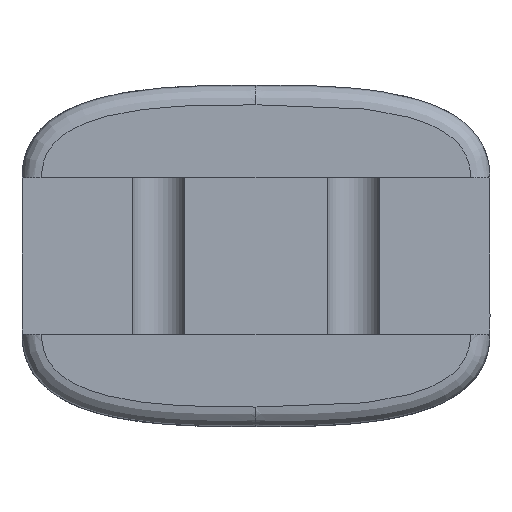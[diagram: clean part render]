
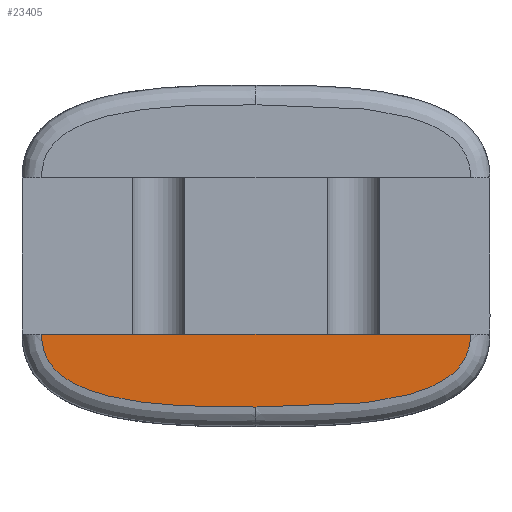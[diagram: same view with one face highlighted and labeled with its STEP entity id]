
A CAD part, top view. The second image highlights one B-rep face of the part: STEP entity #23405.
In plain terms, the highlighted planar face has unit normal (0, 0, 1).
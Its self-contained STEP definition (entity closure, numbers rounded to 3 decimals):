
#26 = CARTESIAN_POINT ( 'NONE',  ( 20.801, 31.551, 43.202 ) ) ;
#451 = CARTESIAN_POINT ( 'NONE',  ( 0., 27.499, 43.202 ) ) ;
#1950 = CARTESIAN_POINT ( 'NONE',  ( -21.732, 33.176, 43.202 ) ) ;
#2040 = CARTESIAN_POINT ( 'NONE',  ( -16.279, 28.948, 43.202 ) ) ;
#2088 = CARTESIAN_POINT ( 'NONE',  ( 14.739, 28.511, 43.202 ) ) ;
#2142 = CARTESIAN_POINT ( 'NONE',  ( 0., 27.499, 43.202 ) ) ;
#2191 = CARTESIAN_POINT ( 'NONE',  ( 21.277, 32.198, 43.202 ) ) ;
#2438 = DIRECTION ( 'NONE',  ( -1., 0., 0. ) ) ;
#3012 = VERTEX_POINT ( 'NONE', #7062 ) ;
#3443 = VERTEX_POINT ( 'NONE', #12315 ) ;
#3592 = CARTESIAN_POINT ( 'NONE',  ( 1.058, 27.499, 43.202 ) ) ;
#3852 = EDGE_CURVE ( 'NONE', #23555, #3012, #21742, .T. ) ;
#4094 = CARTESIAN_POINT ( 'NONE',  ( -21.416, 32.439, 43.202 ) ) ;
#4183 = CARTESIAN_POINT ( 'NONE',  ( -14.744, 28.533, 43.202 ) ) ;
#4212 = ORIENTED_EDGE ( 'NONE', *, *, #3852, .T. ) ;
#4233 = CARTESIAN_POINT ( 'NONE',  ( 16.773, 29.108, 43.202 ) ) ;
#4324 = CARTESIAN_POINT ( 'NONE',  ( 21.634, 32.908, 43.202 ) ) ;
#6139 = ORIENTED_EDGE ( 'NONE', *, *, #10730, .T. ) ;
#6226 = CARTESIAN_POINT ( 'NONE',  ( -20.983, 31.773, 43.202 ) ) ;
#6318 = CARTESIAN_POINT ( 'NONE',  ( -13.187, 28.218, 43.202 ) ) ;
#6364 = CARTESIAN_POINT ( 'NONE',  ( 18.248, 29.703, 43.202 ) ) ;
#6469 = CARTESIAN_POINT ( 'NONE',  ( 21.938, 33.923, 43.202 ) ) ;
#7062 = CARTESIAN_POINT ( 'NONE',  ( 22., 34.963, 43.202 ) ) ;
#8382 = CARTESIAN_POINT ( 'NONE',  ( -20.446, 31.177, 43.202 ) ) ;
#8429 = CARTESIAN_POINT ( 'NONE',  ( 4.23, 27.513, 43.202 ) ) ;
#8481 = CARTESIAN_POINT ( 'NONE',  ( -10.573, 27.849, 43.202 ) ) ;
#8525 = CARTESIAN_POINT ( 'NONE',  ( 19.18, 30.217, 43.202 ) ) ;
#8616 = CARTESIAN_POINT ( 'NONE',  ( 22., 34.963, 43.202 ) ) ;
#10380 = LINE ( 'NONE', #17290, #21672 ) ;
#10497 = CARTESIAN_POINT ( 'NONE',  ( -15.226, 26.597, 43.202 ) ) ;
#10505 = CARTESIAN_POINT ( 'NONE',  ( -19.635, 30.496, 43.202 ) ) ;
#10548 = CARTESIAN_POINT ( 'NONE',  ( 7.399, 27.61, 43.202 ) ) ;
#10597 = CARTESIAN_POINT ( 'NONE',  ( -7.408, 27.611, 43.202 ) ) ;
#10646 = CARTESIAN_POINT ( 'NONE',  ( 19.837, 30.661, 43.202 ) ) ;
#10730 = EDGE_CURVE ( 'NONE', #3443, #23555, #14412, .T. ) ;
#12315 = CARTESIAN_POINT ( 'NONE',  ( -22., 34.963, 43.202 ) ) ;
#12542 = CARTESIAN_POINT ( 'NONE',  ( -21.997, 34.441, 43.202 ) ) ;
#12623 = DIRECTION ( 'NONE',  ( 0., 0., -1. ) ) ;
#12631 = CARTESIAN_POINT ( 'NONE',  ( -18.248, 29.703, 43.202 ) ) ;
#12677 = CARTESIAN_POINT ( 'NONE',  ( 10.562, 27.848, 43.202 ) ) ;
#12727 = CARTESIAN_POINT ( 'NONE',  ( -4.234, 27.513, 43.202 ) ) ;
#12778 = CARTESIAN_POINT ( 'NONE',  ( 20.438, 31.17, 43.202 ) ) ;
#14412 = B_SPLINE_CURVE_WITH_KNOTS ( 'NONE', 3,
 ( #26937, #12542, #14667, #1950, #16812, #4094, #18938, #6226, #21078, #8382, #23216, #10505, #25352, #12631, #27480, #14761, #2040, #16904, #4183, #19027, #6318, #21165, #8481, #23307, #10597, #25445, #12727, #27573, #14846, #2142 ),
 .UNSPECIFIED., .F., .F.,
 ( 4, 2, 2, 2, 2, 2, 2, 2, 2, 2, 2, 2, 2, 2, 4 ),
 ( 0., 0.002, 0.002, 0.003, 0.004, 0.005, 0.006, 0.008, 0.009, 0.011, 0.013, 0.016, 0.019, 0.022, 0.025 ),
 .UNSPECIFIED. ) ;
#14667 = CARTESIAN_POINT ( 'NONE',  ( -21.938, 33.929, 43.202 ) ) ;
#14761 = CARTESIAN_POINT ( 'NONE',  ( -16.78, 29.111, 43.202 ) ) ;
#14802 = CARTESIAN_POINT ( 'NONE',  ( 13.705, 28.3, 43.202 ) ) ;
#14846 = CARTESIAN_POINT ( 'NONE',  ( -1.059, 27.499, 43.202 ) ) ;
#14897 = CARTESIAN_POINT ( 'NONE',  ( 20.972, 31.758, 43.202 ) ) ;
#16474 = ORIENTED_EDGE ( 'NONE', *, *, #26401, .T. ) ;
#16812 = CARTESIAN_POINT ( 'NONE',  ( -21.641, 32.923, 43.202 ) ) ;
#16904 = CARTESIAN_POINT ( 'NONE',  ( -15.261, 28.659, 43.202 ) ) ;
#16951 = CARTESIAN_POINT ( 'NONE',  ( 16.266, 28.944, 43.202 ) ) ;
#17049 = CARTESIAN_POINT ( 'NONE',  ( 21.41, 32.428, 43.202 ) ) ;
#17290 = CARTESIAN_POINT ( 'NONE',  ( -15.226, 34.963, 43.202 ) ) ;
#18678 = AXIS2_PLACEMENT_3D ( 'NONE', #10497, #12623, #27474 ) ;
#18938 = CARTESIAN_POINT ( 'NONE',  ( -21.284, 32.209, 43.202 ) ) ;
#19027 = CARTESIAN_POINT ( 'NONE',  ( -13.708, 28.313, 43.202 ) ) ;
#19042 = FACE_OUTER_BOUND ( 'NONE', #21986, .T. ) ;
#19071 = CARTESIAN_POINT ( 'NONE',  ( 17.764, 29.488, 43.202 ) ) ;
#19164 = CARTESIAN_POINT ( 'NONE',  ( 21.727, 33.159, 43.202 ) ) ;
#21078 = CARTESIAN_POINT ( 'NONE',  ( -20.814, 31.566, 43.202 ) ) ;
#21124 = CARTESIAN_POINT ( 'NONE',  ( 2.115, 27.496, 43.202 ) ) ;
#21165 = CARTESIAN_POINT ( 'NONE',  ( -11.622, 27.968, 43.202 ) ) ;
#21217 = CARTESIAN_POINT ( 'NONE',  ( 18.949, 30.081, 43.202 ) ) ;
#21305 = CARTESIAN_POINT ( 'NONE',  ( 21.997, 34.439, 43.202 ) ) ;
#21672 = VECTOR ( 'NONE', #2438, 1000. ) ;
#21742 = B_SPLINE_CURVE_WITH_KNOTS ( 'NONE', 3,
 ( #24758, #3592, #21124, #8429, #23263, #10548, #25405, #12677, #27530, #14802, #2088, #16951, #4233, #19071, #6364, #21217, #8525, #23351, #10646, #25491, #12778, #26, #14897, #2191, #17049, #4324, #19164, #6469, #21305, #8616 ),
 .UNSPECIFIED., .F., .F.,
 ( 4, 2, 2, 2, 2, 2, 2, 2, 2, 2, 2, 2, 2, 2, 4 ),
 ( 0., 0.003, 0.006, 0.01, 0.013, 0.016, 0.017, 0.019, 0.02, 0.021, 0.021, 0.022, 0.023, 0.024, 0.025 ),
 .UNSPECIFIED. ) ;
#21986 = EDGE_LOOP ( 'NONE', ( #4212, #16474, #6139 ) ) ;
#23216 = CARTESIAN_POINT ( 'NONE',  ( -20.25, 30.998, 43.202 ) ) ;
#23263 = CARTESIAN_POINT ( 'NONE',  ( 5.286, 27.532, 43.202 ) ) ;
#23307 = CARTESIAN_POINT ( 'NONE',  ( -8.466, 27.67, 43.202 ) ) ;
#23351 = CARTESIAN_POINT ( 'NONE',  ( 19.623, 30.507, 43.202 ) ) ;
#23405 = ADVANCED_FACE ( 'NONE', ( #19042 ), #25255, .F. ) ;
#23555 = VERTEX_POINT ( 'NONE', #451 ) ;
#24758 = CARTESIAN_POINT ( 'NONE',  ( 0., 27.499, 43.202 ) ) ;
#25255 = PLANE ( 'NONE',  #18678 ) ;
#25352 = CARTESIAN_POINT ( 'NONE',  ( -19.186, 30.208, 43.202 ) ) ;
#25405 = CARTESIAN_POINT ( 'NONE',  ( 8.454, 27.669, 43.202 ) ) ;
#25445 = CARTESIAN_POINT ( 'NONE',  ( -5.292, 27.532, 43.202 ) ) ;
#25491 = CARTESIAN_POINT ( 'NONE',  ( 20.244, 30.992, 43.202 ) ) ;
#26401 = EDGE_CURVE ( 'NONE', #3012, #3443, #10380, .T. ) ;
#26937 = CARTESIAN_POINT ( 'NONE',  ( -22., 34.963, 43.202 ) ) ;
#27474 = DIRECTION ( 'NONE',  ( 0., 1., 0. ) ) ;
#27480 = CARTESIAN_POINT ( 'NONE',  ( -17.765, 29.489, 43.202 ) ) ;
#27530 = CARTESIAN_POINT ( 'NONE',  ( 11.617, 27.968, 43.202 ) ) ;
#27573 = CARTESIAN_POINT ( 'NONE',  ( -2.117, 27.496, 43.202 ) ) ;
